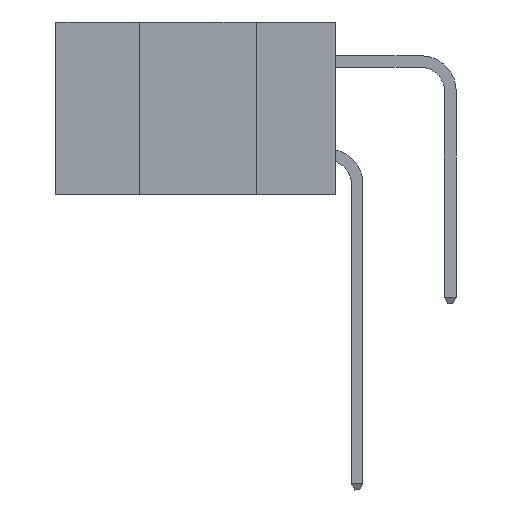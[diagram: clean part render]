
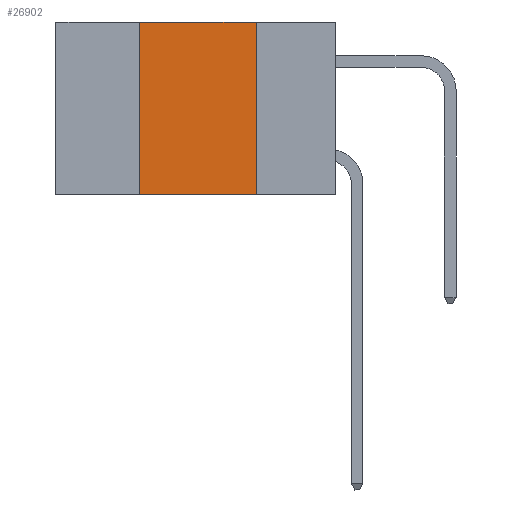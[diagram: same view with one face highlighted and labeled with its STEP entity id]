
A CAD part, left-side view. The second image highlights one B-rep face of the part: STEP entity #26902.
In plain terms, the highlighted planar face has unit normal (-1, 0, 0).
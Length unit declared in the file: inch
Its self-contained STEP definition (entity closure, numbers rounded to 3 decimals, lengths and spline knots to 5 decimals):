
#23 = FACE_OUTER_BOUND ( 'NONE', #24079, .T. ) ;
#217 = VERTEX_POINT ( 'NONE', #17478 ) ;
#1261 = EDGE_CURVE ( 'NONE', #22295, #2440, #3366, .T. ) ;
#2027 = EDGE_CURVE ( 'NONE', #217, #14568, #18952, .T. ) ;
#2183 = AXIS2_PLACEMENT_3D ( 'NONE', #18036, #5036, #20089 ) ;
#2440 = VERTEX_POINT ( 'NONE', #17476 ) ;
#2793 = PLANE ( 'NONE',  #2183 ) ;
#3212 = LINE ( 'NONE', #20570, #14845 ) ;
#3366 = LINE ( 'NONE', #15376, #25427 ) ;
#5036 = DIRECTION ( 'NONE',  ( 1., 0., 0. ) ) ;
#5598 = VECTOR ( 'NONE', #7466, 39.37008 ) ;
#7466 = DIRECTION ( 'NONE',  ( 0., 0., 1. ) ) ;
#7469 = VECTOR ( 'NONE', #16108, 39.37008 ) ;
#8434 = ORIENTED_EDGE ( 'NONE', *, *, #15779, .F. ) ;
#11726 = CARTESIAN_POINT ( 'NONE',  ( 0., 0.42, 0. ) ) ;
#14568 = VERTEX_POINT ( 'NONE', #24450 ) ;
#14845 = VECTOR ( 'NONE', #22642, 39.37008 ) ;
#15195 = EDGE_CURVE ( 'NONE', #2440, #14568, #3212, .T. ) ;
#15376 = CARTESIAN_POINT ( 'NONE',  ( 0., 0.6, 0. ) ) ;
#15779 = EDGE_CURVE ( 'NONE', #217, #22295, #17184, .T. ) ;
#16108 = DIRECTION ( 'NONE',  ( 0., -1., 0. ) ) ;
#16464 = CARTESIAN_POINT ( 'NONE',  ( 0., 0.6, -0.37 ) ) ;
#17184 = LINE ( 'NONE', #11726, #5598 ) ;
#17476 = CARTESIAN_POINT ( 'NONE',  ( 0., 0.17, 0. ) ) ;
#17478 = CARTESIAN_POINT ( 'NONE',  ( 0., 0.42, -0.37 ) ) ;
#18036 = CARTESIAN_POINT ( 'NONE',  ( 0., 0.6, 0. ) ) ;
#18952 = LINE ( 'NONE', #16464, #7469 ) ;
#20089 = DIRECTION ( 'NONE',  ( 0., 0., -1. ) ) ;
#20570 = CARTESIAN_POINT ( 'NONE',  ( 0., 0.17, 0. ) ) ;
#20875 = DIRECTION ( 'NONE',  ( 0., -1., 0. ) ) ;
#21141 = ORIENTED_EDGE ( 'NONE', *, *, #2027, .T. ) ;
#21310 = ORIENTED_EDGE ( 'NONE', *, *, #15195, .F. ) ;
#22295 = VERTEX_POINT ( 'NONE', #22601 ) ;
#22601 = CARTESIAN_POINT ( 'NONE',  ( 0., 0.42, 0. ) ) ;
#22642 = DIRECTION ( 'NONE',  ( 0., 0., -1. ) ) ;
#24079 = EDGE_LOOP ( 'NONE', ( #21310, #25637, #8434, #21141 ) ) ;
#24450 = CARTESIAN_POINT ( 'NONE',  ( 0., 0.17, -0.37 ) ) ;
#25427 = VECTOR ( 'NONE', #20875, 39.37008 ) ;
#25637 = ORIENTED_EDGE ( 'NONE', *, *, #1261, .F. ) ;
#26902 = ADVANCED_FACE ( 'NONE', ( #23 ), #2793, .F. ) ;
